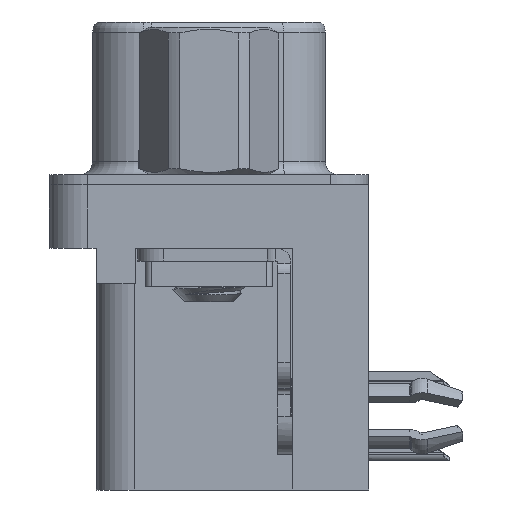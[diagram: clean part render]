
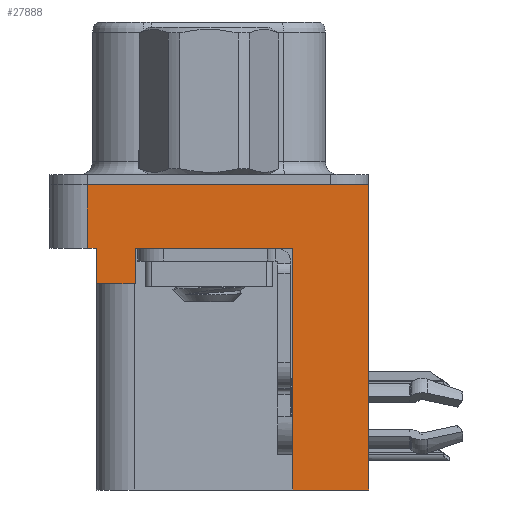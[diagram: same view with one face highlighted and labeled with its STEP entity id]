
A CAD part, left-side view. The second image highlights one B-rep face of the part: STEP entity #27888.
In plain terms, the highlighted planar face has unit normal (-1, 0, 0).
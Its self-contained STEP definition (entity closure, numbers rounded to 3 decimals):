
#362 = CARTESIAN_POINT ( 'NONE',  ( -3., -6.275, 0. ) ) ;
#1134 = CARTESIAN_POINT ( 'NONE',  ( -3., 4.425, -3.9 ) ) ;
#1288 = EDGE_CURVE ( 'NONE', #15901, #4432, #15787, .T. ) ;
#1446 = EDGE_CURVE ( 'NONE', #8368, #15901, #13167, .T. ) ;
#1840 = CARTESIAN_POINT ( 'NONE',  ( -3., -3.295, -12. ) ) ;
#1848 = CARTESIAN_POINT ( 'NONE',  ( -3., 4.425, -3.9 ) ) ;
#2101 = VECTOR ( 'NONE', #5810, 1000. ) ;
#2337 = LINE ( 'NONE', #1848, #7323 ) ;
#2546 = VERTEX_POINT ( 'NONE', #3189 ) ;
#2809 = EDGE_CURVE ( 'NONE', #6026, #26903, #17840, .T. ) ;
#3189 = CARTESIAN_POINT ( 'NONE',  ( -3., 4.775, 0. ) ) ;
#3495 = VERTEX_POINT ( 'NONE', #13508 ) ;
#3612 = ORIENTED_EDGE ( 'NONE', *, *, #12892, .T. ) ;
#4150 = FACE_OUTER_BOUND ( 'NONE', #27981, .T. ) ;
#4332 = EDGE_CURVE ( 'NONE', #8368, #3495, #21708, .T. ) ;
#4359 = LINE ( 'NONE', #362, #12973 ) ;
#4425 = VECTOR ( 'NONE', #20436, 1000. ) ;
#4432 = VERTEX_POINT ( 'NONE', #9141 ) ;
#5810 = DIRECTION ( 'NONE',  ( 0., 0., 1. ) ) ;
#6026 = VERTEX_POINT ( 'NONE', #10386 ) ;
#6071 = LINE ( 'NONE', #1134, #17614 ) ;
#6299 = VECTOR ( 'NONE', #11673, 1000. ) ;
#6366 = ORIENTED_EDGE ( 'NONE', *, *, #20191, .F. ) ;
#6616 = EDGE_CURVE ( 'NONE', #12502, #12886, #6071, .T. ) ;
#6879 = CARTESIAN_POINT ( 'NONE',  ( -3., 4.775, -2.5 ) ) ;
#7322 = ORIENTED_EDGE ( 'NONE', *, *, #11071, .F. ) ;
#7323 = VECTOR ( 'NONE', #22258, 1000. ) ;
#8054 = PLANE ( 'NONE',  #8793 ) ;
#8232 = DIRECTION ( 'NONE',  ( 0., 0., 1. ) ) ;
#8368 = VERTEX_POINT ( 'NONE', #19272 ) ;
#8708 = VECTOR ( 'NONE', #14368, 1000. ) ;
#8793 = AXIS2_PLACEMENT_3D ( 'NONE', #21949, #10490, #24147 ) ;
#8886 = LINE ( 'NONE', #24223, #11424 ) ;
#9141 = CARTESIAN_POINT ( 'NONE',  ( -3., -3.295, -2.5 ) ) ;
#10346 = CARTESIAN_POINT ( 'NONE',  ( -3., -3.295, -12. ) ) ;
#10386 = CARTESIAN_POINT ( 'NONE',  ( -3., 2.895, -3.9 ) ) ;
#10490 = DIRECTION ( 'NONE',  ( -1., 0., 0. ) ) ;
#11071 = EDGE_CURVE ( 'NONE', #2546, #3495, #4359, .T. ) ;
#11256 = LINE ( 'NONE', #26200, #8708 ) ;
#11424 = VECTOR ( 'NONE', #14900, 1000. ) ;
#11673 = DIRECTION ( 'NONE',  ( 0., 0., 1. ) ) ;
#11707 = DIRECTION ( 'NONE',  ( 0., 0., 1. ) ) ;
#12059 = ORIENTED_EDGE ( 'NONE', *, *, #2809, .T. ) ;
#12241 = CARTESIAN_POINT ( 'NONE',  ( -3., 4.425, -2.5 ) ) ;
#12502 = VERTEX_POINT ( 'NONE', #26734 ) ;
#12729 = ORIENTED_EDGE ( 'NONE', *, *, #29515, .F. ) ;
#12886 = VERTEX_POINT ( 'NONE', #12241 ) ;
#12892 = EDGE_CURVE ( 'NONE', #14083, #12886, #11256, .T. ) ;
#12973 = VECTOR ( 'NONE', #20939, 1000. ) ;
#13167 = LINE ( 'NONE', #1840, #28987 ) ;
#13508 = CARTESIAN_POINT ( 'NONE',  ( -3., -6.275, 0. ) ) ;
#13771 = ORIENTED_EDGE ( 'NONE', *, *, #4332, .T. ) ;
#14083 = VERTEX_POINT ( 'NONE', #6879 ) ;
#14368 = DIRECTION ( 'NONE',  ( 0., -1., 0. ) ) ;
#14900 = DIRECTION ( 'NONE',  ( 0., -1., 0. ) ) ;
#15787 = LINE ( 'NONE', #10346, #2101 ) ;
#15901 = VERTEX_POINT ( 'NONE', #23993 ) ;
#17027 = VECTOR ( 'NONE', #11707, 1000. ) ;
#17614 = VECTOR ( 'NONE', #8232, 1000. ) ;
#17711 = CARTESIAN_POINT ( 'NONE',  ( -3., -6.275, -2.5 ) ) ;
#17840 = LINE ( 'NONE', #23124, #6299 ) ;
#18186 = CARTESIAN_POINT ( 'NONE',  ( -3., 2.895, -2.5 ) ) ;
#18307 = ORIENTED_EDGE ( 'NONE', *, *, #1446, .F. ) ;
#18603 = ORIENTED_EDGE ( 'NONE', *, *, #6616, .F. ) ;
#19272 = CARTESIAN_POINT ( 'NONE',  ( -3., -6.275, -12. ) ) ;
#20191 = EDGE_CURVE ( 'NONE', #6026, #12502, #2337, .T. ) ;
#20436 = DIRECTION ( 'NONE',  ( 0., 0., 1. ) ) ;
#20690 = CARTESIAN_POINT ( 'NONE',  ( -3., 4.775, -2.5 ) ) ;
#20939 = DIRECTION ( 'NONE',  ( 0., -1., 0. ) ) ;
#21708 = LINE ( 'NONE', #17711, #4425 ) ;
#21949 = CARTESIAN_POINT ( 'NONE',  ( -3., -6.275, -2.5 ) ) ;
#22258 = DIRECTION ( 'NONE',  ( 0., 1., 0. ) ) ;
#23124 = CARTESIAN_POINT ( 'NONE',  ( -3., 2.895, -3.9 ) ) ;
#23993 = CARTESIAN_POINT ( 'NONE',  ( -3., -3.295, -12. ) ) ;
#24147 = DIRECTION ( 'NONE',  ( 0., 0., 1. ) ) ;
#24223 = CARTESIAN_POINT ( 'NONE',  ( -3., -6.275, -2.5 ) ) ;
#24810 = EDGE_CURVE ( 'NONE', #26903, #4432, #8886, .T. ) ;
#24877 = DIRECTION ( 'NONE',  ( 0., 1., 0. ) ) ;
#26200 = CARTESIAN_POINT ( 'NONE',  ( -3., -6.275, -2.5 ) ) ;
#26287 = ORIENTED_EDGE ( 'NONE', *, *, #24810, .T. ) ;
#26734 = CARTESIAN_POINT ( 'NONE',  ( -3., 4.425, -3.9 ) ) ;
#26903 = VERTEX_POINT ( 'NONE', #18186 ) ;
#27888 = ADVANCED_FACE ( 'NONE', ( #4150 ), #8054, .T. ) ;
#27981 = EDGE_LOOP ( 'NONE', ( #7322, #12729, #3612, #18603, #6366, #12059, #26287, #29191, #18307, #13771 ) ) ;
#28987 = VECTOR ( 'NONE', #24877, 1000. ) ;
#29185 = LINE ( 'NONE', #20690, #17027 ) ;
#29191 = ORIENTED_EDGE ( 'NONE', *, *, #1288, .F. ) ;
#29515 = EDGE_CURVE ( 'NONE', #14083, #2546, #29185, .T. ) ;
